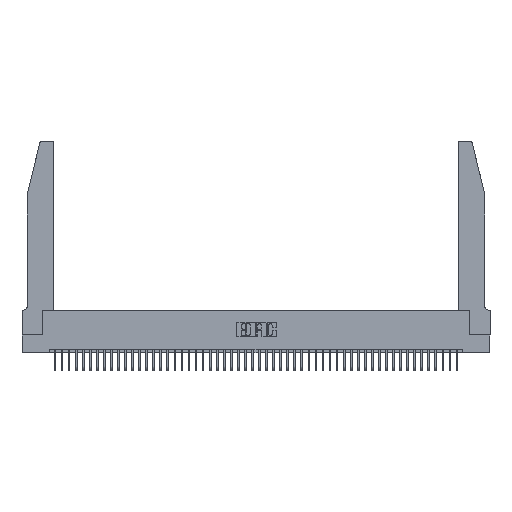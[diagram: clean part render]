
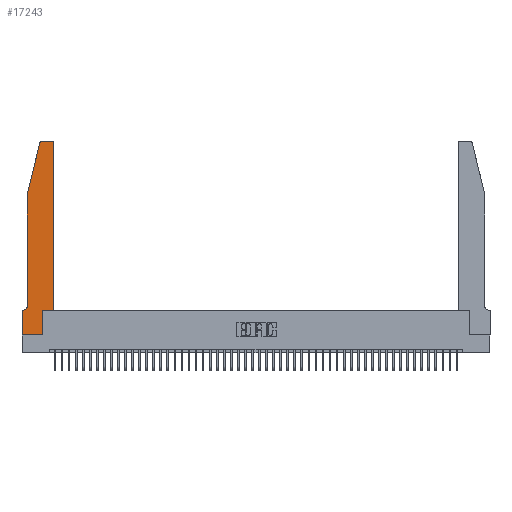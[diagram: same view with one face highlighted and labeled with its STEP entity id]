
A CAD part, top view. The second image highlights one B-rep face of the part: STEP entity #17243.
In plain terms, the highlighted planar face has unit normal (0, 0, 1).
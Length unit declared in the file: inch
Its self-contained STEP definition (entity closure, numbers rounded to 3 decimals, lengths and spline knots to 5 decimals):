
#316 = ORIENTED_EDGE ( 'NONE', *, *, #31162, .T. ) ;
#318 = FACE_OUTER_BOUND ( 'NONE', #21428, .T. ) ;
#727 = DIRECTION ( 'NONE',  ( 1., 0., 0. ) ) ;
#777 = CARTESIAN_POINT ( 'NONE',  ( 0.2865, 0.35, 0.37 ) ) ;
#1039 = VECTOR ( 'NONE', #39985, 39.37008 ) ;
#1098 = CARTESIAN_POINT ( 'NONE',  ( 0.0055, 0.35, 0.37 ) ) ;
#1537 = CARTESIAN_POINT ( 'NONE',  ( 0.2865, 0.35, 0.37 ) ) ;
#3817 = LINE ( 'NONE', #21530, #40790 ) ;
#3907 = DIRECTION ( 'NONE',  ( 0., 0., -1. ) ) ;
#5225 = VERTEX_POINT ( 'NONE', #1098 ) ;
#5942 = ORIENTED_EDGE ( 'NONE', *, *, #30480, .T. ) ;
#6711 = AXIS2_PLACEMENT_3D ( 'NONE', #25455, #3907, #29035 ) ;
#7212 = EDGE_CURVE ( 'NONE', #13618, #43008, #27581, .T. ) ;
#7239 = VECTOR ( 'NONE', #8776, 39.37008 ) ;
#7260 = CARTESIAN_POINT ( 'NONE',  ( 0.25487, 2.72718, 0.37 ) ) ;
#7345 = CARTESIAN_POINT ( 'NONE',  ( 0.4205, 2.72, 0.37 ) ) ;
#7346 = ORIENTED_EDGE ( 'NONE', *, *, #36374, .T. ) ;
#7849 = VERTEX_POINT ( 'NONE', #36202 ) ;
#7866 = CARTESIAN_POINT ( 'NONE',  ( 0.2605, 2.75, 0.37 ) ) ;
#8380 = CARTESIAN_POINT ( 'NONE',  ( 0.0755, 2., 0.37 ) ) ;
#8593 = EDGE_CURVE ( 'NONE', #7849, #19360, #3817, .T. ) ;
#8776 = DIRECTION ( 'NONE',  ( 0., 1., 0. ) ) ;
#9891 = ORIENTED_EDGE ( 'NONE', *, *, #21525, .T. ) ;
#10986 = DIRECTION ( 'NONE',  ( 1., 0., 0. ) ) ;
#11268 = DIRECTION ( 'NONE',  ( 1., 0., 0. ) ) ;
#13618 = VERTEX_POINT ( 'NONE', #25950 ) ;
#13900 = LINE ( 'NONE', #36646, #31802 ) ;
#13995 = VECTOR ( 'NONE', #34679, 39.37008 ) ;
#14972 = CARTESIAN_POINT ( 'NONE',  ( 0., 0.35, 0.37 ) ) ;
#15036 = LINE ( 'NONE', #43619, #32891 ) ;
#15567 = AXIS2_PLACEMENT_3D ( 'NONE', #15994, #40937, #19619 ) ;
#15675 = EDGE_CURVE ( 'NONE', #35069, #22023, #19072, .T. ) ;
#15994 = CARTESIAN_POINT ( 'NONE',  ( 0.284, 2.72, 0.37 ) ) ;
#17091 = CARTESIAN_POINT ( 'NONE',  ( 0.0755, 2., 0.37 ) ) ;
#17206 = CIRCLE ( 'NONE', #6711, 0.07 ) ;
#17243 = ADVANCED_FACE ( 'NONE', ( #318 ), #36330, .T. ) ;
#17972 = LINE ( 'NONE', #8380, #27486 ) ;
#18581 = DIRECTION ( 'NONE',  ( 0., 0., 1. ) ) ;
#18640 = CARTESIAN_POINT ( 'NONE',  ( 0.0755, 2., 0.37 ) ) ;
#19072 = LINE ( 'NONE', #18640, #1039 ) ;
#19360 = VERTEX_POINT ( 'NONE', #31000 ) ;
#19619 = DIRECTION ( 'NONE',  ( 1., 0., 0. ) ) ;
#20055 = EDGE_CURVE ( 'NONE', #5225, #20676, #23565, .T. ) ;
#20166 = ORIENTED_EDGE ( 'NONE', *, *, #32347, .T. ) ;
#20676 = VERTEX_POINT ( 'NONE', #41368 ) ;
#21428 = EDGE_LOOP ( 'NONE', ( #33752, #31464, #42356, #5942, #26796, #23634, #20166, #38005, #316, #7346, #23870, #9891 ) ) ;
#21525 = EDGE_CURVE ( 'NONE', #19360, #26426, #39032, .T. ) ;
#21530 = CARTESIAN_POINT ( 'NONE',  ( 0.4505, 0.35, 0.37 ) ) ;
#22023 = VERTEX_POINT ( 'NONE', #17091 ) ;
#22869 = AXIS2_PLACEMENT_3D ( 'NONE', #7345, #32425, #10986 ) ;
#23565 = LINE ( 'NONE', #34515, #13995 ) ;
#23634 = ORIENTED_EDGE ( 'NONE', *, *, #20055, .T. ) ;
#23870 = ORIENTED_EDGE ( 'NONE', *, *, #8593, .T. ) ;
#25455 = CARTESIAN_POINT ( 'NONE',  ( 0.0055, 0.42, 0.37 ) ) ;
#25950 = CARTESIAN_POINT ( 'NONE',  ( 0., 0., 0.37 ) ) ;
#25958 = VERTEX_POINT ( 'NONE', #45487 ) ;
#26426 = VERTEX_POINT ( 'NONE', #44842 ) ;
#26796 = ORIENTED_EDGE ( 'NONE', *, *, #42564, .T. ) ;
#27486 = VECTOR ( 'NONE', #33406, 39.37008 ) ;
#27581 = LINE ( 'NONE', #36090, #34757 ) ;
#29035 = DIRECTION ( 'NONE',  ( -1., 0., 0. ) ) ;
#30480 = EDGE_CURVE ( 'NONE', #22023, #25958, #17972, .T. ) ;
#31000 = CARTESIAN_POINT ( 'NONE',  ( 0.4505, 2.72, 0.37 ) ) ;
#31025 = VERTEX_POINT ( 'NONE', #777 ) ;
#31162 = EDGE_CURVE ( 'NONE', #43008, #31025, #36937, .T. ) ;
#31464 = ORIENTED_EDGE ( 'NONE', *, *, #34692, .T. ) ;
#31802 = VECTOR ( 'NONE', #40244, 39.37008 ) ;
#32347 = EDGE_CURVE ( 'NONE', #20676, #13618, #13900, .T. ) ;
#32425 = DIRECTION ( 'NONE',  ( 0., 0., 1. ) ) ;
#32891 = VECTOR ( 'NONE', #727, 39.37008 ) ;
#33138 = VECTOR ( 'NONE', #43516, 39.37008 ) ;
#33406 = DIRECTION ( 'NONE',  ( 0., -1., 0. ) ) ;
#33752 = ORIENTED_EDGE ( 'NONE', *, *, #45696, .T. ) ;
#33852 = VERTEX_POINT ( 'NONE', #38367 ) ;
#34515 = CARTESIAN_POINT ( 'NONE',  ( 0.0755, 0.35, 0.37 ) ) ;
#34679 = DIRECTION ( 'NONE',  ( -1., 0., 0. ) ) ;
#34692 = EDGE_CURVE ( 'NONE', #33852, #35069, #46036, .T. ) ;
#34757 = VECTOR ( 'NONE', #11268, 39.37008 ) ;
#35069 = VERTEX_POINT ( 'NONE', #7260 ) ;
#36090 = CARTESIAN_POINT ( 'NONE',  ( 0., 0., 0.37 ) ) ;
#36202 = CARTESIAN_POINT ( 'NONE',  ( 0.4505, 0.35, 0.37 ) ) ;
#36330 = PLANE ( 'NONE',  #41525 ) ;
#36374 = EDGE_CURVE ( 'NONE', #31025, #7849, #15036, .T. ) ;
#36646 = CARTESIAN_POINT ( 'NONE',  ( 0., 0., 0.37 ) ) ;
#36937 = LINE ( 'NONE', #1537, #7239 ) ;
#38005 = ORIENTED_EDGE ( 'NONE', *, *, #7212, .T. ) ;
#38367 = CARTESIAN_POINT ( 'NONE',  ( 0.284, 2.75, 0.37 ) ) ;
#39032 = CIRCLE ( 'NONE', #22869, 0.03 ) ;
#39985 = DIRECTION ( 'NONE',  ( -0.239, -0.971, 0. ) ) ;
#40244 = DIRECTION ( 'NONE',  ( 0., -1., 0. ) ) ;
#40790 = VECTOR ( 'NONE', #42837, 39.37008 ) ;
#40937 = DIRECTION ( 'NONE',  ( 0., 0., 1. ) ) ;
#41368 = CARTESIAN_POINT ( 'NONE',  ( 0., 0.35, 0.37 ) ) ;
#41525 = AXIS2_PLACEMENT_3D ( 'NONE', #14972, #18581, #43509 ) ;
#42356 = ORIENTED_EDGE ( 'NONE', *, *, #15675, .T. ) ;
#42476 = CARTESIAN_POINT ( 'NONE',  ( 0.2865, 0., 0.37 ) ) ;
#42564 = EDGE_CURVE ( 'NONE', #25958, #5225, #17206, .T. ) ;
#42618 = LINE ( 'NONE', #7866, #33138 ) ;
#42837 = DIRECTION ( 'NONE',  ( 0., 1., 0. ) ) ;
#43008 = VERTEX_POINT ( 'NONE', #42476 ) ;
#43509 = DIRECTION ( 'NONE',  ( 1., 0., 0. ) ) ;
#43516 = DIRECTION ( 'NONE',  ( -1., 0., 0. ) ) ;
#43619 = CARTESIAN_POINT ( 'NONE',  ( 0.4505, 0.35, 0.37 ) ) ;
#44842 = CARTESIAN_POINT ( 'NONE',  ( 0.4205, 2.75, 0.37 ) ) ;
#45487 = CARTESIAN_POINT ( 'NONE',  ( 0.0755, 0.42, 0.37 ) ) ;
#45696 = EDGE_CURVE ( 'NONE', #26426, #33852, #42618, .T. ) ;
#46036 = CIRCLE ( 'NONE', #15567, 0.03 ) ;
